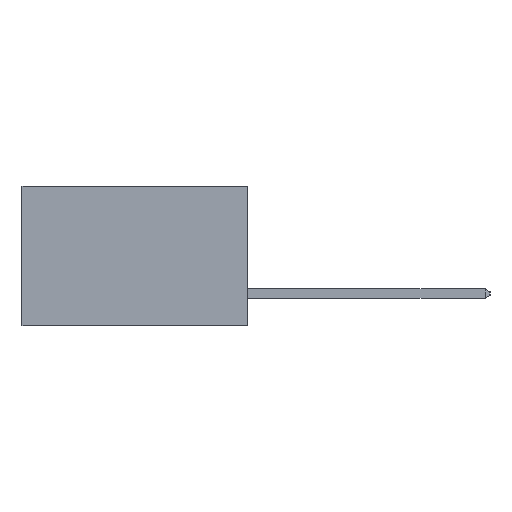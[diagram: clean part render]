
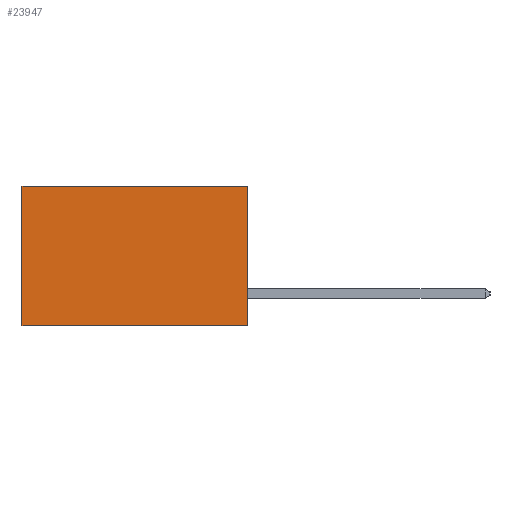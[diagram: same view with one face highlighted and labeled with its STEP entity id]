
A CAD part, left-side view. The second image highlights one B-rep face of the part: STEP entity #23947.
In plain terms, the highlighted planar face has unit normal (-1, 0, 0).
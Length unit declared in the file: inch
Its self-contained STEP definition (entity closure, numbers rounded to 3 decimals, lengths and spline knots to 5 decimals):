
#539 = VERTEX_POINT ( 'NONE', #871 ) ;
#871 = CARTESIAN_POINT ( 'NONE',  ( 0.298, 0.6, 0. ) ) ;
#2941 = LINE ( 'NONE', #3058, #12731 ) ;
#3058 = CARTESIAN_POINT ( 'NONE',  ( 0.298, 0., 0. ) ) ;
#3486 = DIRECTION ( 'NONE',  ( 0., 0., -1. ) ) ;
#4294 = DIRECTION ( 'NONE',  ( 0., 1., 0. ) ) ;
#5658 = VECTOR ( 'NONE', #15642, 39.37008 ) ;
#7012 = CARTESIAN_POINT ( 'NONE',  ( 0.298, 0., 0. ) ) ;
#7952 = VERTEX_POINT ( 'NONE', #11465 ) ;
#8652 = AXIS2_PLACEMENT_3D ( 'NONE', #19115, #15267, #3486 ) ;
#9319 = ORIENTED_EDGE ( 'NONE', *, *, #21079, .F. ) ;
#9387 = VECTOR ( 'NONE', #4294, 39.37008 ) ;
#9787 = VERTEX_POINT ( 'NONE', #11912 ) ;
#10634 = ORIENTED_EDGE ( 'NONE', *, *, #10782, .T. ) ;
#10782 = EDGE_CURVE ( 'NONE', #15911, #539, #2941, .T. ) ;
#11465 = CARTESIAN_POINT ( 'NONE',  ( 0.298, 0.6, -0.37 ) ) ;
#11912 = CARTESIAN_POINT ( 'NONE',  ( 0.298, 0., -0.37 ) ) ;
#12731 = VECTOR ( 'NONE', #24551, 39.37008 ) ;
#13589 = ORIENTED_EDGE ( 'NONE', *, *, #21537, .T. ) ;
#13641 = CARTESIAN_POINT ( 'NONE',  ( 0.298, 0.6, 0. ) ) ;
#15267 = DIRECTION ( 'NONE',  ( 1., 0., 0. ) ) ;
#15388 = FACE_OUTER_BOUND ( 'NONE', #17255, .T. ) ;
#15500 = CARTESIAN_POINT ( 'NONE',  ( 0.298, 0., 0. ) ) ;
#15642 = DIRECTION ( 'NONE',  ( 0., 0., -1. ) ) ;
#15911 = VERTEX_POINT ( 'NONE', #7012 ) ;
#16110 = CARTESIAN_POINT ( 'NONE',  ( 0.298, 0., -0.37 ) ) ;
#17010 = VECTOR ( 'NONE', #23190, 39.37008 ) ;
#17255 = EDGE_LOOP ( 'NONE', ( #13589, #9319, #19102, #10634 ) ) ;
#18233 = LINE ( 'NONE', #15500, #17010 ) ;
#19102 = ORIENTED_EDGE ( 'NONE', *, *, #22846, .F. ) ;
#19115 = CARTESIAN_POINT ( 'NONE',  ( 0.298, 0., 0. ) ) ;
#21079 = EDGE_CURVE ( 'NONE', #9787, #7952, #23154, .T. ) ;
#21344 = LINE ( 'NONE', #13641, #5658 ) ;
#21537 = EDGE_CURVE ( 'NONE', #539, #7952, #21344, .T. ) ;
#22846 = EDGE_CURVE ( 'NONE', #15911, #9787, #18233, .T. ) ;
#22984 = PLANE ( 'NONE',  #8652 ) ;
#23154 = LINE ( 'NONE', #16110, #9387 ) ;
#23190 = DIRECTION ( 'NONE',  ( 0., 0., -1. ) ) ;
#23947 = ADVANCED_FACE ( 'NONE', ( #15388 ), #22984, .F. ) ;
#24551 = DIRECTION ( 'NONE',  ( 0., 1., 0. ) ) ;
